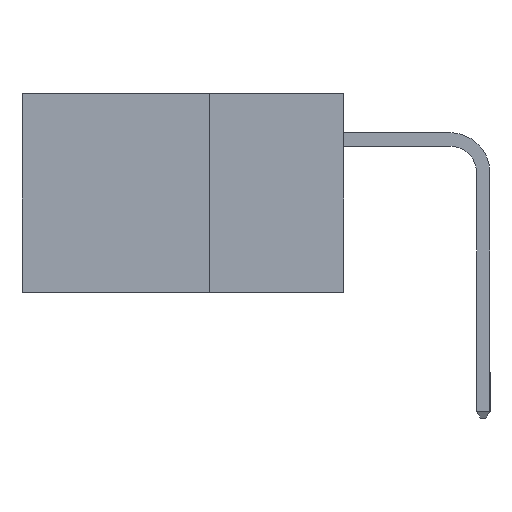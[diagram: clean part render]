
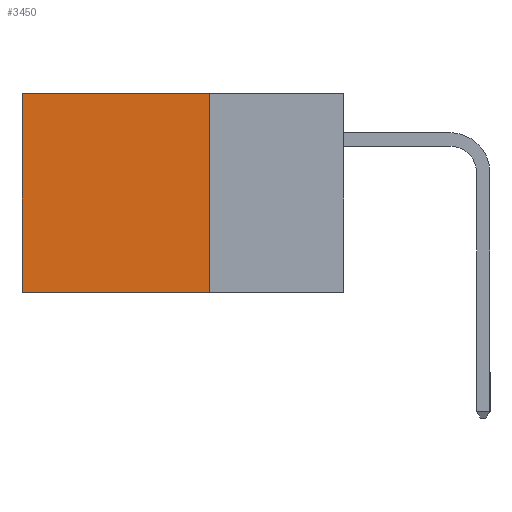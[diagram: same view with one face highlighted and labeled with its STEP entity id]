
A CAD part, left-side view. The second image highlights one B-rep face of the part: STEP entity #3450.
In plain terms, the highlighted planar face has unit normal (-1, 0, 0).
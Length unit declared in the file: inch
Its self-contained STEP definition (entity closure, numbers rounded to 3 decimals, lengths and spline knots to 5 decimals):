
#4 = DIRECTION ( 'NONE',  ( 0., 0., -1. ) ) ;
#163 = ORIENTED_EDGE ( 'NONE', *, *, #8447, .T. ) ;
#279 = DIRECTION ( 'NONE',  ( 0., 1., 0. ) ) ;
#809 = EDGE_CURVE ( 'NONE', #12404, #10863, #3973, .T. ) ;
#1282 = CARTESIAN_POINT ( 'NONE',  ( 0.298, 0.6, 0. ) ) ;
#1606 = ORIENTED_EDGE ( 'NONE', *, *, #809, .F. ) ;
#2689 = LINE ( 'NONE', #14165, #4256 ) ;
#3161 = DIRECTION ( 'NONE',  ( 1., 0., 0. ) ) ;
#3367 = LINE ( 'NONE', #1282, #8772 ) ;
#3450 = ADVANCED_FACE ( 'NONE', ( #3522 ), #13004, .F. ) ;
#3522 = FACE_OUTER_BOUND ( 'NONE', #12625, .T. ) ;
#3973 = LINE ( 'NONE', #8063, #9002 ) ;
#4256 = VECTOR ( 'NONE', #9361, 39.37008 ) ;
#4367 = CARTESIAN_POINT ( 'NONE',  ( 0.298, 0.6, 0. ) ) ;
#6089 = EDGE_CURVE ( 'NONE', #12404, #9392, #11045, .T. ) ;
#6265 = CARTESIAN_POINT ( 'NONE',  ( 0.298, 0.25, 0. ) ) ;
#7633 = EDGE_CURVE ( 'NONE', #10863, #12730, #2689, .T. ) ;
#8063 = CARTESIAN_POINT ( 'NONE',  ( 0.298, 0.25, 0. ) ) ;
#8170 = ORIENTED_EDGE ( 'NONE', *, *, #7633, .F. ) ;
#8331 = CARTESIAN_POINT ( 'NONE',  ( 0.298, 0.25, 0. ) ) ;
#8447 = EDGE_CURVE ( 'NONE', #9392, #12730, #3367, .T. ) ;
#8675 = CARTESIAN_POINT ( 'NONE',  ( 0.298, 0.25, 0. ) ) ;
#8772 = VECTOR ( 'NONE', #4, 39.37008 ) ;
#8790 = CARTESIAN_POINT ( 'NONE',  ( 0.298, 0.25, -0.37 ) ) ;
#9002 = VECTOR ( 'NONE', #15477, 39.37008 ) ;
#9361 = DIRECTION ( 'NONE',  ( 0., 1., 0. ) ) ;
#9392 = VERTEX_POINT ( 'NONE', #4367 ) ;
#10863 = VERTEX_POINT ( 'NONE', #8790 ) ;
#11045 = LINE ( 'NONE', #8675, #15857 ) ;
#11966 = DIRECTION ( 'NONE',  ( 0., 0., -1. ) ) ;
#12404 = VERTEX_POINT ( 'NONE', #6265 ) ;
#12625 = EDGE_LOOP ( 'NONE', ( #163, #8170, #1606, #13498 ) ) ;
#12730 = VERTEX_POINT ( 'NONE', #14416 ) ;
#13004 = PLANE ( 'NONE',  #15902 ) ;
#13498 = ORIENTED_EDGE ( 'NONE', *, *, #6089, .T. ) ;
#14165 = CARTESIAN_POINT ( 'NONE',  ( 0.298, 0.25, -0.37 ) ) ;
#14416 = CARTESIAN_POINT ( 'NONE',  ( 0.298, 0.6, -0.37 ) ) ;
#15477 = DIRECTION ( 'NONE',  ( 0., 0., -1. ) ) ;
#15857 = VECTOR ( 'NONE', #279, 39.37008 ) ;
#15902 = AXIS2_PLACEMENT_3D ( 'NONE', #8331, #3161, #11966 ) ;
